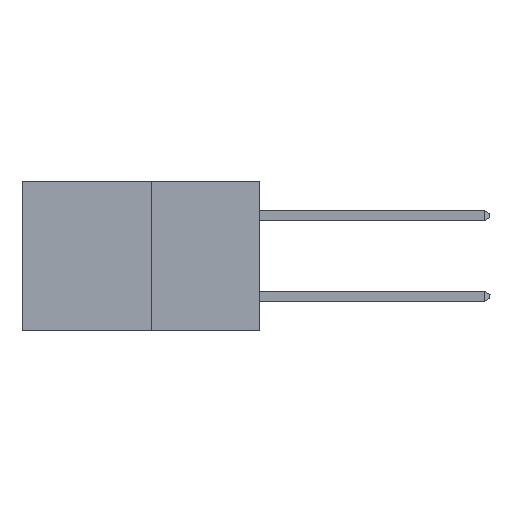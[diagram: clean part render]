
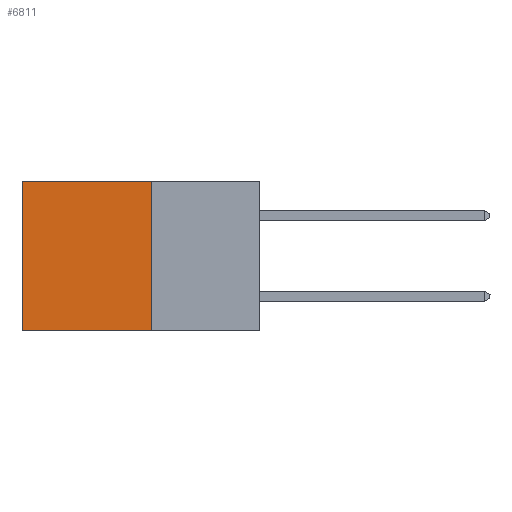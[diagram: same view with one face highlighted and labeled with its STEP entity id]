
A CAD part, left-side view. The second image highlights one B-rep face of the part: STEP entity #6811.
In plain terms, the highlighted planar face has unit normal (-1, 0, 0).
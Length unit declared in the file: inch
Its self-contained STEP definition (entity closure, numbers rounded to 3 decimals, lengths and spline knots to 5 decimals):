
#8 = LINE ( 'NONE', #10623, #7463 ) ;
#343 = CARTESIAN_POINT ( 'NONE',  ( 0.277, 0.27, 0. ) ) ;
#361 = DIRECTION ( 'NONE',  ( 0., 1., 0. ) ) ;
#1147 = VERTEX_POINT ( 'NONE', #22071 ) ;
#1560 = ORIENTED_EDGE ( 'NONE', *, *, #9951, .F. ) ;
#1838 = LINE ( 'NONE', #2178, #20957 ) ;
#2178 = CARTESIAN_POINT ( 'NONE',  ( 0.277, 0.27, -0.37 ) ) ;
#3284 = DIRECTION ( 'NONE',  ( 0., 0., -1. ) ) ;
#4692 = EDGE_CURVE ( 'NONE', #17281, #12089, #14921, .T. ) ;
#5110 = VECTOR ( 'NONE', #15849, 39.37008 ) ;
#5418 = PLANE ( 'NONE',  #20466 ) ;
#6004 = CARTESIAN_POINT ( 'NONE',  ( 0.277, 0.59, 0. ) ) ;
#6599 = DIRECTION ( 'NONE',  ( 0., 0., -1. ) ) ;
#6811 = ADVANCED_FACE ( 'NONE', ( #7879 ), #5418, .F. ) ;
#7258 = CARTESIAN_POINT ( 'NONE',  ( 0.277, 0.59, -0.37 ) ) ;
#7463 = VECTOR ( 'NONE', #3284, 39.37008 ) ;
#7879 = FACE_OUTER_BOUND ( 'NONE', #9861, .T. ) ;
#7928 = ORIENTED_EDGE ( 'NONE', *, *, #9213, .T. ) ;
#8949 = VECTOR ( 'NONE', #12407, 39.37008 ) ;
#9213 = EDGE_CURVE ( 'NONE', #12089, #18456, #13860, .T. ) ;
#9861 = EDGE_LOOP ( 'NONE', ( #7928, #20095, #1560, #22411 ) ) ;
#9951 = EDGE_CURVE ( 'NONE', #17281, #1147, #8, .T. ) ;
#10574 = CARTESIAN_POINT ( 'NONE',  ( 0.277, 0.59, -0.37 ) ) ;
#10623 = CARTESIAN_POINT ( 'NONE',  ( 0.277, 0.27, -0.37 ) ) ;
#12089 = VERTEX_POINT ( 'NONE', #6004 ) ;
#12407 = DIRECTION ( 'NONE',  ( 0., 0., -1. ) ) ;
#13186 = DIRECTION ( 'NONE',  ( 1., 0., 0. ) ) ;
#13860 = LINE ( 'NONE', #10574, #8949 ) ;
#14921 = LINE ( 'NONE', #15560, #5110 ) ;
#15560 = CARTESIAN_POINT ( 'NONE',  ( 0.277, 0.27, 0. ) ) ;
#15849 = DIRECTION ( 'NONE',  ( 0., 1., 0. ) ) ;
#17281 = VERTEX_POINT ( 'NONE', #343 ) ;
#18456 = VERTEX_POINT ( 'NONE', #7258 ) ;
#20095 = ORIENTED_EDGE ( 'NONE', *, *, #21602, .F. ) ;
#20466 = AXIS2_PLACEMENT_3D ( 'NONE', #20835, #13186, #6599 ) ;
#20835 = CARTESIAN_POINT ( 'NONE',  ( 0.277, 0.27, -0.37 ) ) ;
#20957 = VECTOR ( 'NONE', #361, 39.37008 ) ;
#21602 = EDGE_CURVE ( 'NONE', #1147, #18456, #1838, .T. ) ;
#22071 = CARTESIAN_POINT ( 'NONE',  ( 0.277, 0.27, -0.37 ) ) ;
#22411 = ORIENTED_EDGE ( 'NONE', *, *, #4692, .T. ) ;
